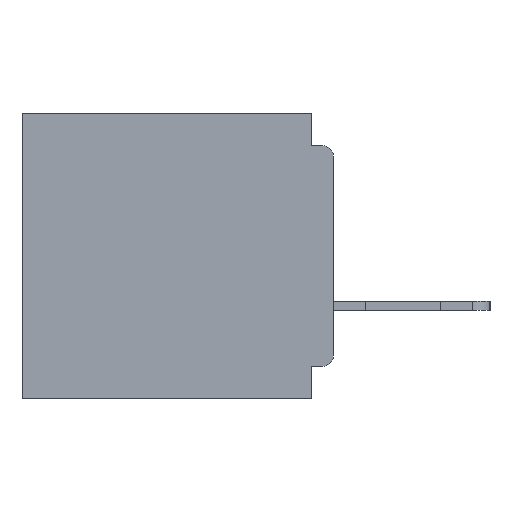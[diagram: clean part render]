
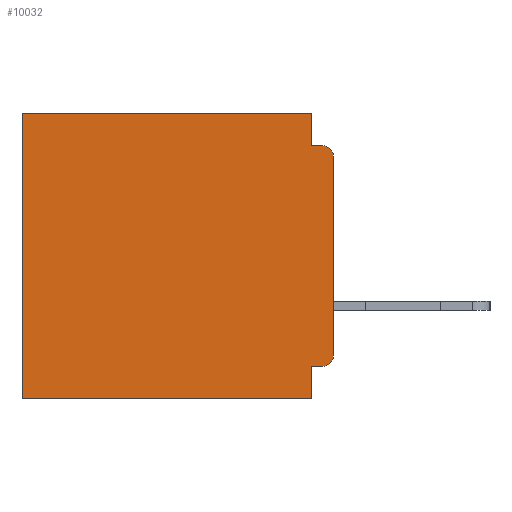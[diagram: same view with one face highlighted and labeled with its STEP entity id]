
A CAD part, left-side view. The second image highlights one B-rep face of the part: STEP entity #10032.
In plain terms, the highlighted planar face has unit normal (-1, 0, 0).
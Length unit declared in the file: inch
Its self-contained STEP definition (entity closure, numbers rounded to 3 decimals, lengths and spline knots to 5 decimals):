
#233 = AXIS2_PLACEMENT_3D ( 'NONE', #27782, #7036, #31286 ) ;
#426 = CARTESIAN_POINT ( 'NONE',  ( 0.3, 0., -0.34 ) ) ;
#1043 = VECTOR ( 'NONE', #9888, 39.37008 ) ;
#1049 = EDGE_CURVE ( 'NONE', #9307, #8597, #17306, .T. ) ;
#1998 = LINE ( 'NONE', #2682, #28679 ) ;
#2682 = CARTESIAN_POINT ( 'NONE',  ( 0.3, 0.031, -0.4 ) ) ;
#2764 = DIRECTION ( 'NONE',  ( 0., 0., -1. ) ) ;
#3695 = EDGE_CURVE ( 'NONE', #44857, #9277, #32837, .T. ) ;
#4305 = EDGE_CURVE ( 'NONE', #6161, #22597, #38949, .T. ) ;
#4818 = VECTOR ( 'NONE', #4907, 39.37008 ) ;
#4907 = DIRECTION ( 'NONE',  ( 0., 0., -1. ) ) ;
#5158 = VECTOR ( 'NONE', #25354, 39.37008 ) ;
#5287 = ORIENTED_EDGE ( 'NONE', *, *, #4305, .F. ) ;
#5320 = CARTESIAN_POINT ( 'NONE',  ( 0.3, 0.015, -0.355 ) ) ;
#5530 = VERTEX_POINT ( 'NONE', #15332 ) ;
#5768 = EDGE_CURVE ( 'NONE', #25066, #44857, #12832, .T. ) ;
#6161 = VERTEX_POINT ( 'NONE', #35447 ) ;
#6180 = EDGE_LOOP ( 'NONE', ( #10292, #35486, #30495, #28591, #18287, #43317, #5287, #10506, #22052, #18258 ) ) ;
#6388 = CARTESIAN_POINT ( 'NONE',  ( 0.3, 0., 0. ) ) ;
#6821 = DIRECTION ( 'NONE',  ( 0., 1., 0. ) ) ;
#7036 = DIRECTION ( 'NONE',  ( -1., 0., 0. ) ) ;
#7339 = EDGE_CURVE ( 'NONE', #29016, #9277, #38195, .T. ) ;
#8597 = VERTEX_POINT ( 'NONE', #426 ) ;
#9058 = CARTESIAN_POINT ( 'NONE',  ( 0.3, 0.031, 0. ) ) ;
#9277 = VERTEX_POINT ( 'NONE', #42875 ) ;
#9307 = VERTEX_POINT ( 'NONE', #5320 ) ;
#9678 = CARTESIAN_POINT ( 'NONE',  ( 0.3, 0.031, -0.355 ) ) ;
#9840 = CARTESIAN_POINT ( 'NONE',  ( 0.3, 0.031, 0. ) ) ;
#9888 = DIRECTION ( 'NONE',  ( 0., 1., 0. ) ) ;
#10032 = ADVANCED_FACE ( 'NONE', ( #34727 ), #37535, .F. ) ;
#10292 = ORIENTED_EDGE ( 'NONE', *, *, #18000, .F. ) ;
#10506 = ORIENTED_EDGE ( 'NONE', *, *, #23949, .F. ) ;
#10774 = CARTESIAN_POINT ( 'NONE',  ( 0.3, 0., -0.06 ) ) ;
#11349 = CARTESIAN_POINT ( 'NONE',  ( 0.3, 0., -0.4 ) ) ;
#12832 = LINE ( 'NONE', #9840, #29103 ) ;
#13247 = DIRECTION ( 'NONE',  ( 0., 0., -1. ) ) ;
#14850 = DIRECTION ( 'NONE',  ( 0., 1., 0. ) ) ;
#15332 = CARTESIAN_POINT ( 'NONE',  ( 0.3, 0.437, 0. ) ) ;
#16803 = DIRECTION ( 'NONE',  ( 1., 0., 0. ) ) ;
#16920 = DIRECTION ( 'NONE',  ( -1., 0., 0. ) ) ;
#17296 = EDGE_CURVE ( 'NONE', #9307, #42540, #29119, .T. ) ;
#17306 = CIRCLE ( 'NONE', #28662, 0.015 ) ;
#18000 = EDGE_CURVE ( 'NONE', #29016, #8597, #44698, .T. ) ;
#18258 = ORIENTED_EDGE ( 'NONE', *, *, #1049, .T. ) ;
#18287 = ORIENTED_EDGE ( 'NONE', *, *, #28000, .T. ) ;
#19890 = VECTOR ( 'NONE', #6821, 39.37008 ) ;
#20134 = CARTESIAN_POINT ( 'NONE',  ( 0.3, 0.437, -0.4 ) ) ;
#20562 = VECTOR ( 'NONE', #14850, 39.37008 ) ;
#20673 = DIRECTION ( 'NONE',  ( 0., 0., -1. ) ) ;
#22052 = ORIENTED_EDGE ( 'NONE', *, *, #17296, .F. ) ;
#22207 = LINE ( 'NONE', #25720, #4818 ) ;
#22597 = VERTEX_POINT ( 'NONE', #20134 ) ;
#23292 = CARTESIAN_POINT ( 'NONE',  ( 0.3, 0.031, -0.045 ) ) ;
#23691 = EDGE_CURVE ( 'NONE', #5530, #22597, #22207, .T. ) ;
#23949 = EDGE_CURVE ( 'NONE', #42540, #6161, #1998, .T. ) ;
#25066 = VERTEX_POINT ( 'NONE', #9058 ) ;
#25354 = DIRECTION ( 'NONE',  ( 0., -1., 0. ) ) ;
#25720 = CARTESIAN_POINT ( 'NONE',  ( 0.3, 0.437, -0.4 ) ) ;
#27561 = CARTESIAN_POINT ( 'NONE',  ( 0.3, 0., -0.355 ) ) ;
#27782 = CARTESIAN_POINT ( 'NONE',  ( 0.3, 0.015, -0.06 ) ) ;
#28000 = EDGE_CURVE ( 'NONE', #25066, #5530, #39077, .T. ) ;
#28591 = ORIENTED_EDGE ( 'NONE', *, *, #5768, .F. ) ;
#28662 = AXIS2_PLACEMENT_3D ( 'NONE', #36864, #16920, #20673 ) ;
#28679 = VECTOR ( 'NONE', #13247, 39.37008 ) ;
#29016 = VERTEX_POINT ( 'NONE', #10774 ) ;
#29103 = VECTOR ( 'NONE', #2764, 39.37008 ) ;
#29119 = LINE ( 'NONE', #27561, #19890 ) ;
#30495 = ORIENTED_EDGE ( 'NONE', *, *, #3695, .F. ) ;
#31286 = DIRECTION ( 'NONE',  ( 0., 0., -1. ) ) ;
#32155 = CARTESIAN_POINT ( 'NONE',  ( 0.3, 0., -0.045 ) ) ;
#32837 = LINE ( 'NONE', #32155, #5158 ) ;
#34727 = FACE_OUTER_BOUND ( 'NONE', #6180, .T. ) ;
#34954 = CARTESIAN_POINT ( 'NONE',  ( 0.3, 0., -0.4 ) ) ;
#35447 = CARTESIAN_POINT ( 'NONE',  ( 0.3, 0.031, -0.4 ) ) ;
#35486 = ORIENTED_EDGE ( 'NONE', *, *, #7339, .T. ) ;
#35527 = VECTOR ( 'NONE', #38394, 39.37008 ) ;
#36864 = CARTESIAN_POINT ( 'NONE',  ( 0.3, 0.015, -0.34 ) ) ;
#37535 = PLANE ( 'NONE',  #39019 ) ;
#38195 = CIRCLE ( 'NONE', #233, 0.015 ) ;
#38394 = DIRECTION ( 'NONE',  ( 0., 0., -1. ) ) ;
#38949 = LINE ( 'NONE', #11349, #20562 ) ;
#39019 = AXIS2_PLACEMENT_3D ( 'NONE', #40826, #16803, #40983 ) ;
#39077 = LINE ( 'NONE', #6388, #1043 ) ;
#40826 = CARTESIAN_POINT ( 'NONE',  ( 0.3, 0., -0.4 ) ) ;
#40983 = DIRECTION ( 'NONE',  ( 0., 0., -1. ) ) ;
#42540 = VERTEX_POINT ( 'NONE', #9678 ) ;
#42875 = CARTESIAN_POINT ( 'NONE',  ( 0.3, 0.015, -0.045 ) ) ;
#43317 = ORIENTED_EDGE ( 'NONE', *, *, #23691, .T. ) ;
#44698 = LINE ( 'NONE', #34954, #35527 ) ;
#44857 = VERTEX_POINT ( 'NONE', #23292 ) ;
